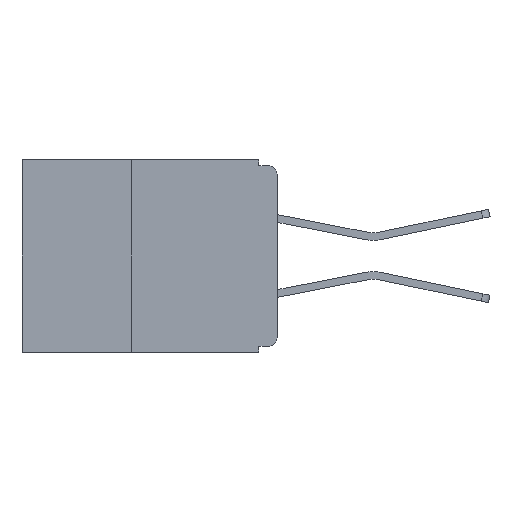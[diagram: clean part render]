
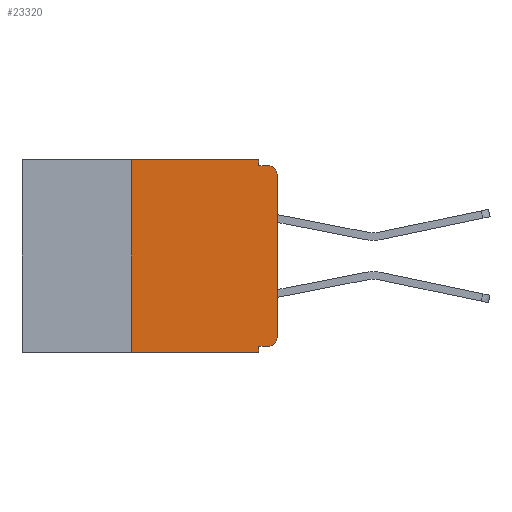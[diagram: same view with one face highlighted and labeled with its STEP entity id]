
A CAD part, left-side view. The second image highlights one B-rep face of the part: STEP entity #23320.
In plain terms, the highlighted planar face has unit normal (-1, 0, 0).
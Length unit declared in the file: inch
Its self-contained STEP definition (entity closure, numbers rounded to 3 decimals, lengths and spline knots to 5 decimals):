
#1120 = DIRECTION ( 'NONE',  ( 0., -1., 0. ) ) ;
#2207 = CIRCLE ( 'NONE', #29130, 0.015 ) ;
#2336 = LINE ( 'NONE', #30789, #14835 ) ;
#2641 = CARTESIAN_POINT ( 'NONE',  ( 0., 0.015, -0.32 ) ) ;
#2915 = CARTESIAN_POINT ( 'NONE',  ( 0., 0., 0. ) ) ;
#2928 = CARTESIAN_POINT ( 'NONE',  ( 0., 0.437, 0. ) ) ;
#2967 = VERTEX_POINT ( 'NONE', #26110 ) ;
#3271 = ORIENTED_EDGE ( 'NONE', *, *, #3504, .F. ) ;
#3504 = EDGE_CURVE ( 'NONE', #22445, #31087, #18964, .T. ) ;
#4161 = VECTOR ( 'NONE', #25182, 39.37008 ) ;
#4966 = VERTEX_POINT ( 'NONE', #4977 ) ;
#4977 = CARTESIAN_POINT ( 'NONE',  ( 0., 0.25, -0.33 ) ) ;
#5014 = VERTEX_POINT ( 'NONE', #2641 ) ;
#5194 = LINE ( 'NONE', #2915, #24190 ) ;
#5236 = CARTESIAN_POINT ( 'NONE',  ( 0., 0.031, 0. ) ) ;
#5574 = PLANE ( 'NONE',  #5949 ) ;
#5737 = EDGE_CURVE ( 'NONE', #5014, #17640, #23956, .T. ) ;
#5801 = VECTOR ( 'NONE', #1120, 39.37008 ) ;
#5949 = AXIS2_PLACEMENT_3D ( 'NONE', #2928, #22902, #8123 ) ;
#6163 = EDGE_LOOP ( 'NONE', ( #6852, #20791, #8453, #10011, #3271, #17280, #6441, #9601, #16912, #23492 ) ) ;
#6197 = CARTESIAN_POINT ( 'NONE',  ( 0., 0., -0.305 ) ) ;
#6428 = CARTESIAN_POINT ( 'NONE',  ( 0., 0., -0.025 ) ) ;
#6441 = ORIENTED_EDGE ( 'NONE', *, *, #26178, .T. ) ;
#6852 = ORIENTED_EDGE ( 'NONE', *, *, #19844, .T. ) ;
#7968 = CARTESIAN_POINT ( 'NONE',  ( 0., 0., -0.01 ) ) ;
#8123 = DIRECTION ( 'NONE',  ( 0., 0., -1. ) ) ;
#8415 = VERTEX_POINT ( 'NONE', #8653 ) ;
#8453 = ORIENTED_EDGE ( 'NONE', *, *, #20493, .F. ) ;
#8653 = CARTESIAN_POINT ( 'NONE',  ( 0., 0.031, -0.01 ) ) ;
#9202 = DIRECTION ( 'NONE',  ( -1., 0., 0. ) ) ;
#9339 = CARTESIAN_POINT ( 'NONE',  ( 0., 0.015, -0.025 ) ) ;
#9601 = ORIENTED_EDGE ( 'NONE', *, *, #30031, .F. ) ;
#9742 = EDGE_CURVE ( 'NONE', #30147, #23561, #11763, .T. ) ;
#9809 = VECTOR ( 'NONE', #22559, 39.37008 ) ;
#10011 = ORIENTED_EDGE ( 'NONE', *, *, #12330, .F. ) ;
#11172 = DIRECTION ( 'NONE',  ( 0., 0., 1. ) ) ;
#11522 = LINE ( 'NONE', #23212, #29596 ) ;
#11763 = CIRCLE ( 'NONE', #17306, 0.015 ) ;
#11808 = DIRECTION ( 'NONE',  ( 0., 0., -1. ) ) ;
#12330 = EDGE_CURVE ( 'NONE', #31087, #8415, #29433, .T. ) ;
#12581 = VERTEX_POINT ( 'NONE', #6197 ) ;
#12850 = CARTESIAN_POINT ( 'NONE',  ( 0., 0., -0.32 ) ) ;
#14345 = FACE_OUTER_BOUND ( 'NONE', #6163, .T. ) ;
#14835 = VECTOR ( 'NONE', #11172, 39.37008 ) ;
#16912 = ORIENTED_EDGE ( 'NONE', *, *, #5737, .F. ) ;
#17280 = ORIENTED_EDGE ( 'NONE', *, *, #29452, .F. ) ;
#17306 = AXIS2_PLACEMENT_3D ( 'NONE', #9339, #26562, #11808 ) ;
#17640 = VERTEX_POINT ( 'NONE', #31956 ) ;
#17815 = DIRECTION ( 'NONE',  ( 0., 0., 1. ) ) ;
#18425 = DIRECTION ( 'NONE',  ( 0., 0., -1. ) ) ;
#18964 = LINE ( 'NONE', #24652, #5801 ) ;
#19844 = EDGE_CURVE ( 'NONE', #12581, #30147, #5194, .T. ) ;
#19904 = VECTOR ( 'NONE', #25238, 39.37008 ) ;
#20493 = EDGE_CURVE ( 'NONE', #8415, #23561, #25716, .T. ) ;
#20791 = ORIENTED_EDGE ( 'NONE', *, *, #9742, .T. ) ;
#21921 = CARTESIAN_POINT ( 'NONE',  ( 0., 0.437, -0.33 ) ) ;
#22184 = CARTESIAN_POINT ( 'NONE',  ( 0., 0.25, 0. ) ) ;
#22445 = VERTEX_POINT ( 'NONE', #22184 ) ;
#22559 = DIRECTION ( 'NONE',  ( 0., 0., -1. ) ) ;
#22902 = DIRECTION ( 'NONE',  ( 1., 0., 0. ) ) ;
#23212 = CARTESIAN_POINT ( 'NONE',  ( 0., 0.031, -0.33 ) ) ;
#23320 = ADVANCED_FACE ( 'NONE', ( #14345 ), #5574, .F. ) ;
#23492 = ORIENTED_EDGE ( 'NONE', *, *, #23586, .T. ) ;
#23561 = VERTEX_POINT ( 'NONE', #23866 ) ;
#23586 = EDGE_CURVE ( 'NONE', #5014, #12581, #2207, .T. ) ;
#23866 = CARTESIAN_POINT ( 'NONE',  ( 0., 0.015, -0.01 ) ) ;
#23956 = LINE ( 'NONE', #12850, #4161 ) ;
#23979 = CARTESIAN_POINT ( 'NONE',  ( 0., 0.015, -0.305 ) ) ;
#24190 = VECTOR ( 'NONE', #17815, 39.37008 ) ;
#24256 = CARTESIAN_POINT ( 'NONE',  ( 0., 0.031, 0. ) ) ;
#24652 = CARTESIAN_POINT ( 'NONE',  ( 0., 0.437, 0. ) ) ;
#25182 = DIRECTION ( 'NONE',  ( 0., 1., 0. ) ) ;
#25238 = DIRECTION ( 'NONE',  ( 0., -1., 0. ) ) ;
#25716 = LINE ( 'NONE', #7968, #19904 ) ;
#26110 = CARTESIAN_POINT ( 'NONE',  ( 0., 0.031, -0.33 ) ) ;
#26178 = EDGE_CURVE ( 'NONE', #4966, #2967, #31095, .T. ) ;
#26422 = DIRECTION ( 'NONE',  ( 0., 0., -1. ) ) ;
#26562 = DIRECTION ( 'NONE',  ( -1., 0., 0. ) ) ;
#26856 = DIRECTION ( 'NONE',  ( 0., -1., 0. ) ) ;
#27319 = VECTOR ( 'NONE', #26856, 39.37008 ) ;
#29130 = AXIS2_PLACEMENT_3D ( 'NONE', #23979, #9202, #26422 ) ;
#29433 = LINE ( 'NONE', #5236, #9809 ) ;
#29452 = EDGE_CURVE ( 'NONE', #4966, #22445, #2336, .T. ) ;
#29596 = VECTOR ( 'NONE', #18425, 39.37008 ) ;
#30031 = EDGE_CURVE ( 'NONE', #17640, #2967, #11522, .T. ) ;
#30147 = VERTEX_POINT ( 'NONE', #6428 ) ;
#30789 = CARTESIAN_POINT ( 'NONE',  ( 0., 0.25, -0.33 ) ) ;
#31087 = VERTEX_POINT ( 'NONE', #24256 ) ;
#31095 = LINE ( 'NONE', #21921, #27319 ) ;
#31956 = CARTESIAN_POINT ( 'NONE',  ( 0., 0.031, -0.32 ) ) ;
